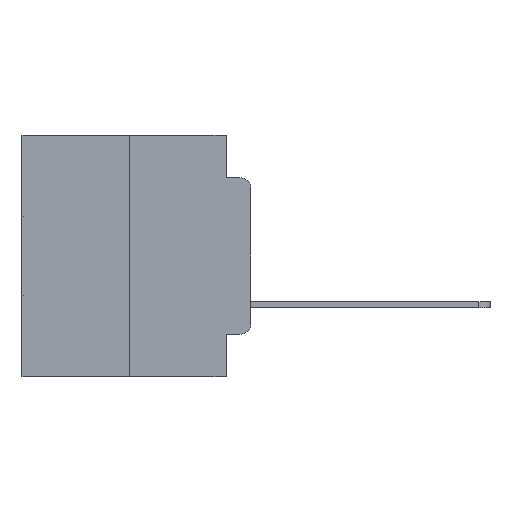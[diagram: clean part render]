
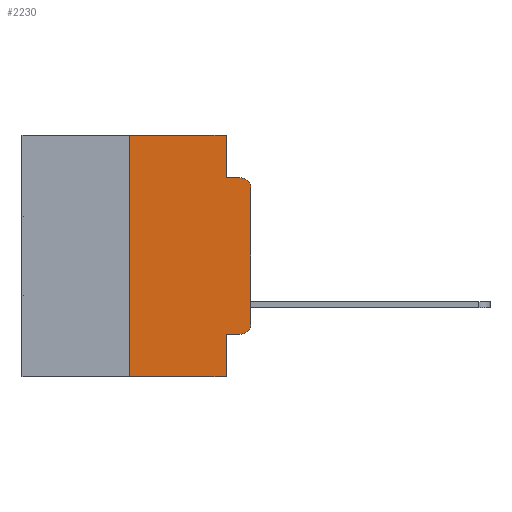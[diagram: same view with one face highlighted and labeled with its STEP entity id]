
A CAD part, left-side view. The second image highlights one B-rep face of the part: STEP entity #2230.
In plain terms, the highlighted planar face has unit normal (-1, 0, 0).
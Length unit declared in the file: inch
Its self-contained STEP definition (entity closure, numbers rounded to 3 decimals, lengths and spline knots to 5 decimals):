
#332 = LINE ( 'NONE', #13255, #6719 ) ;
#369 = CIRCLE ( 'NONE', #6746, 0.02 ) ;
#721 = CARTESIAN_POINT ( 'NONE',  ( 0., 0.02, -0.3915 ) ) ;
#1061 = ORIENTED_EDGE ( 'NONE', *, *, #7944, .F. ) ;
#1097 = EDGE_CURVE ( 'NONE', #14053, #27600, #25990, .T. ) ;
#1444 = CIRCLE ( 'NONE', #11605, 0.02 ) ;
#1836 = ORIENTED_EDGE ( 'NONE', *, *, #1097, .F. ) ;
#2016 = CARTESIAN_POINT ( 'NONE',  ( 0., 0.051, 0. ) ) ;
#2230 = ADVANCED_FACE ( 'NONE', ( #28944 ), #13199, .F. ) ;
#2309 = CARTESIAN_POINT ( 'NONE',  ( 0., 0., 0. ) ) ;
#3016 = ORIENTED_EDGE ( 'NONE', *, *, #8940, .T. ) ;
#3252 = ORIENTED_EDGE ( 'NONE', *, *, #6609, .F. ) ;
#3486 = DIRECTION ( 'NONE',  ( 0., 0., -1. ) ) ;
#3616 = CARTESIAN_POINT ( 'NONE',  ( 0., 0., -0.1085 ) ) ;
#3705 = LINE ( 'NONE', #6383, #16044 ) ;
#3840 = ORIENTED_EDGE ( 'NONE', *, *, #12122, .T. ) ;
#3954 = DIRECTION ( 'NONE',  ( 0., 0., -1. ) ) ;
#4055 = DIRECTION ( 'NONE',  ( 1., 0., 0. ) ) ;
#5279 = VERTEX_POINT ( 'NONE', #12256 ) ;
#5530 = EDGE_CURVE ( 'NONE', #28465, #21359, #1444, .T. ) ;
#5856 = ORIENTED_EDGE ( 'NONE', *, *, #22681, .F. ) ;
#6383 = CARTESIAN_POINT ( 'NONE',  ( 0., 0.473, -0.5 ) ) ;
#6573 = VERTEX_POINT ( 'NONE', #18748 ) ;
#6609 = EDGE_CURVE ( 'NONE', #27600, #22232, #18962, .T. ) ;
#6719 = VECTOR ( 'NONE', #19882, 39.37008 ) ;
#6746 = AXIS2_PLACEMENT_3D ( 'NONE', #8907, #24775, #11293 ) ;
#7941 = LINE ( 'NONE', #10379, #19577 ) ;
#7944 = EDGE_CURVE ( 'NONE', #6573, #14053, #7941, .T. ) ;
#8292 = EDGE_CURVE ( 'NONE', #16550, #22232, #369, .T. ) ;
#8650 = LINE ( 'NONE', #22111, #14306 ) ;
#8907 = CARTESIAN_POINT ( 'NONE',  ( 0., 0.02, -0.1085 ) ) ;
#8940 = EDGE_CURVE ( 'NONE', #20679, #22690, #3705, .T. ) ;
#9378 = CARTESIAN_POINT ( 'NONE',  ( 0., 0.25, -0.5 ) ) ;
#9552 = DIRECTION ( 'NONE',  ( 0., -1., 0. ) ) ;
#10379 = CARTESIAN_POINT ( 'NONE',  ( 0., 0.473, 0. ) ) ;
#11293 = DIRECTION ( 'NONE',  ( 0., 0., -1. ) ) ;
#11605 = AXIS2_PLACEMENT_3D ( 'NONE', #721, #18019, #3486 ) ;
#11971 = CARTESIAN_POINT ( 'NONE',  ( 0., 0.051, -0.0885 ) ) ;
#12122 = EDGE_CURVE ( 'NONE', #5279, #28465, #12750, .T. ) ;
#12142 = DIRECTION ( 'NONE',  ( 0., -1., 0. ) ) ;
#12213 = VECTOR ( 'NONE', #9552, 39.37008 ) ;
#12256 = CARTESIAN_POINT ( 'NONE',  ( 0., 0.051, -0.4115 ) ) ;
#12489 = CARTESIAN_POINT ( 'NONE',  ( 0., 0.02, -0.0885 ) ) ;
#12750 = LINE ( 'NONE', #18898, #29634 ) ;
#12844 = DIRECTION ( 'NONE',  ( 0., -1., 0. ) ) ;
#13199 = PLANE ( 'NONE',  #16753 ) ;
#13255 = CARTESIAN_POINT ( 'NONE',  ( 0., 0.051, 0. ) ) ;
#14053 = VERTEX_POINT ( 'NONE', #2016 ) ;
#14121 = CARTESIAN_POINT ( 'NONE',  ( 0., 0.051, 0. ) ) ;
#14280 = VECTOR ( 'NONE', #18330, 39.37008 ) ;
#14306 = VECTOR ( 'NONE', #26479, 39.37008 ) ;
#14393 = EDGE_LOOP ( 'NONE', ( #15985, #15251, #3252, #1836, #1061, #17521, #3016, #5856, #3840, #26430 ) ) ;
#14729 = EDGE_CURVE ( 'NONE', #21359, #16550, #23748, .T. ) ;
#15251 = ORIENTED_EDGE ( 'NONE', *, *, #8292, .T. ) ;
#15985 = ORIENTED_EDGE ( 'NONE', *, *, #14729, .T. ) ;
#16044 = VECTOR ( 'NONE', #24843, 39.37008 ) ;
#16503 = CARTESIAN_POINT ( 'NONE',  ( 0., 0., -0.3915 ) ) ;
#16550 = VERTEX_POINT ( 'NONE', #3616 ) ;
#16753 = AXIS2_PLACEMENT_3D ( 'NONE', #20075, #4055, #3954 ) ;
#17521 = ORIENTED_EDGE ( 'NONE', *, *, #29900, .F. ) ;
#18019 = DIRECTION ( 'NONE',  ( -1., 0., 0. ) ) ;
#18330 = DIRECTION ( 'NONE',  ( 0., 0., -1. ) ) ;
#18748 = CARTESIAN_POINT ( 'NONE',  ( 0., 0.25, 0. ) ) ;
#18898 = CARTESIAN_POINT ( 'NONE',  ( 0., 0.051, -0.4115 ) ) ;
#18962 = LINE ( 'NONE', #11971, #12213 ) ;
#19413 = CARTESIAN_POINT ( 'NONE',  ( 0., 0.051, -0.0885 ) ) ;
#19577 = VECTOR ( 'NONE', #12844, 39.37008 ) ;
#19882 = DIRECTION ( 'NONE',  ( 0., 0., -1. ) ) ;
#20075 = CARTESIAN_POINT ( 'NONE',  ( 0., 0.473, 0. ) ) ;
#20679 = VERTEX_POINT ( 'NONE', #9378 ) ;
#21359 = VERTEX_POINT ( 'NONE', #16503 ) ;
#21553 = DIRECTION ( 'NONE',  ( 0., 0., 1. ) ) ;
#22111 = CARTESIAN_POINT ( 'NONE',  ( 0., 0.25, 0. ) ) ;
#22232 = VERTEX_POINT ( 'NONE', #12489 ) ;
#22308 = CARTESIAN_POINT ( 'NONE',  ( 0., 0.051, -0.5 ) ) ;
#22386 = VECTOR ( 'NONE', #21553, 39.37008 ) ;
#22681 = EDGE_CURVE ( 'NONE', #5279, #22690, #332, .T. ) ;
#22690 = VERTEX_POINT ( 'NONE', #22308 ) ;
#23748 = LINE ( 'NONE', #2309, #22386 ) ;
#24775 = DIRECTION ( 'NONE',  ( -1., 0., 0. ) ) ;
#24843 = DIRECTION ( 'NONE',  ( 0., -1., 0. ) ) ;
#25990 = LINE ( 'NONE', #14121, #14280 ) ;
#26430 = ORIENTED_EDGE ( 'NONE', *, *, #5530, .T. ) ;
#26479 = DIRECTION ( 'NONE',  ( 0., 0., 1. ) ) ;
#27295 = CARTESIAN_POINT ( 'NONE',  ( 0., 0.02, -0.4115 ) ) ;
#27600 = VERTEX_POINT ( 'NONE', #19413 ) ;
#28465 = VERTEX_POINT ( 'NONE', #27295 ) ;
#28944 = FACE_OUTER_BOUND ( 'NONE', #14393, .T. ) ;
#29634 = VECTOR ( 'NONE', #12142, 39.37008 ) ;
#29900 = EDGE_CURVE ( 'NONE', #20679, #6573, #8650, .T. ) ;
